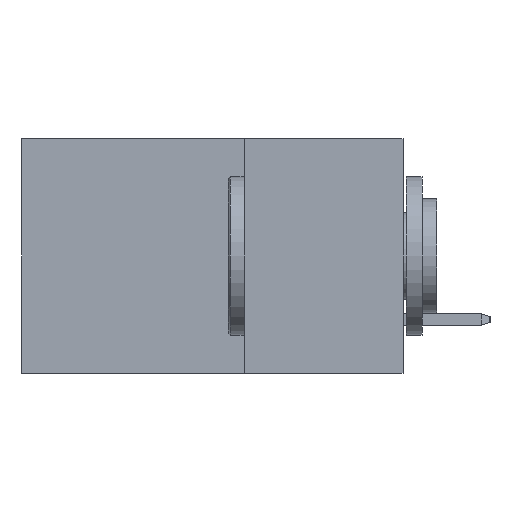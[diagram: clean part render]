
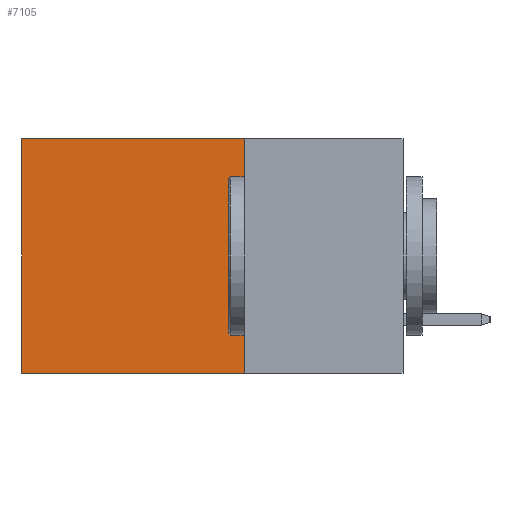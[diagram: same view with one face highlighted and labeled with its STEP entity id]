
A CAD part, left-side view. The second image highlights one B-rep face of the part: STEP entity #7105.
In plain terms, the highlighted planar face has unit normal (-1, 0, 0).
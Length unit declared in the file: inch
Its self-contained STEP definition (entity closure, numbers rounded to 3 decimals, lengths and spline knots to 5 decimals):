
#171 = EDGE_CURVE ( 'NONE', #7540, #2903, #3070, .T. ) ;
#192 = CARTESIAN_POINT ( 'NONE',  ( 0.2875, 0.6, -0.37 ) ) ;
#306 = CARTESIAN_POINT ( 'NONE',  ( 0.2875, 0.25, 0. ) ) ;
#449 = VECTOR ( 'NONE', #2096, 39.37008 ) ;
#736 = ORIENTED_EDGE ( 'NONE', *, *, #7643, .F. ) ;
#918 = EDGE_LOOP ( 'NONE', ( #2620, #10735, #736, #4536 ) ) ;
#1595 = CARTESIAN_POINT ( 'NONE',  ( 0.2875, 0.25, 0. ) ) ;
#1818 = VECTOR ( 'NONE', #4475, 39.37008 ) ;
#2096 = DIRECTION ( 'NONE',  ( 0., 0., -1. ) ) ;
#2617 = CARTESIAN_POINT ( 'NONE',  ( 0.2875, 0.25, -0.37 ) ) ;
#2620 = ORIENTED_EDGE ( 'NONE', *, *, #171, .T. ) ;
#2732 = EDGE_CURVE ( 'NONE', #6873, #2903, #6642, .T. ) ;
#2769 = VECTOR ( 'NONE', #10432, 39.37008 ) ;
#2903 = VERTEX_POINT ( 'NONE', #192 ) ;
#3070 = LINE ( 'NONE', #6005, #449 ) ;
#4475 = DIRECTION ( 'NONE',  ( 0., 1., 0. ) ) ;
#4536 = ORIENTED_EDGE ( 'NONE', *, *, #11757, .T. ) ;
#4614 = DIRECTION ( 'NONE',  ( 0., 0., -1. ) ) ;
#5178 = CARTESIAN_POINT ( 'NONE',  ( 0.2875, 0.25, -0.37 ) ) ;
#5492 = DIRECTION ( 'NONE',  ( 1., 0., 0. ) ) ;
#5977 = VECTOR ( 'NONE', #8900, 39.37008 ) ;
#6005 = CARTESIAN_POINT ( 'NONE',  ( 0.2875, 0.6, 0. ) ) ;
#6642 = LINE ( 'NONE', #2617, #1818 ) ;
#6873 = VERTEX_POINT ( 'NONE', #5178 ) ;
#7105 = ADVANCED_FACE ( 'NONE', ( #10474 ), #11407, .F. ) ;
#7540 = VERTEX_POINT ( 'NONE', #8414 ) ;
#7643 = EDGE_CURVE ( 'NONE', #9754, #6873, #9737, .T. ) ;
#8414 = CARTESIAN_POINT ( 'NONE',  ( 0.2875, 0.6, 0. ) ) ;
#8714 = CARTESIAN_POINT ( 'NONE',  ( 0.2875, 0.25, 0. ) ) ;
#8900 = DIRECTION ( 'NONE',  ( 0., 0., -1. ) ) ;
#9277 = LINE ( 'NONE', #12185, #2769 ) ;
#9737 = LINE ( 'NONE', #8714, #5977 ) ;
#9754 = VERTEX_POINT ( 'NONE', #306 ) ;
#9832 = AXIS2_PLACEMENT_3D ( 'NONE', #1595, #5492, #4614 ) ;
#10432 = DIRECTION ( 'NONE',  ( 0., 1., 0. ) ) ;
#10474 = FACE_OUTER_BOUND ( 'NONE', #918, .T. ) ;
#10735 = ORIENTED_EDGE ( 'NONE', *, *, #2732, .F. ) ;
#11407 = PLANE ( 'NONE',  #9832 ) ;
#11757 = EDGE_CURVE ( 'NONE', #9754, #7540, #9277, .T. ) ;
#12185 = CARTESIAN_POINT ( 'NONE',  ( 0.2875, 0.25, 0. ) ) ;
